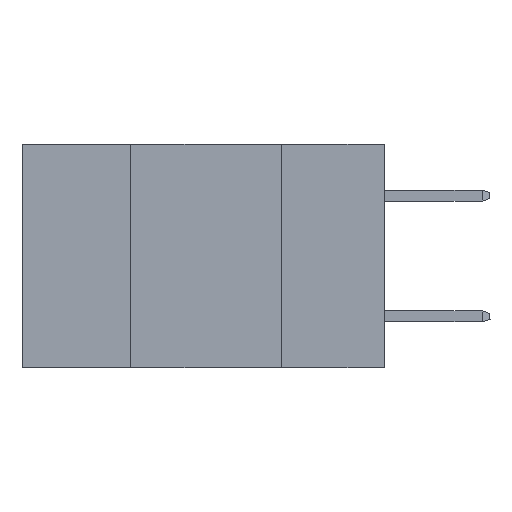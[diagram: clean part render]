
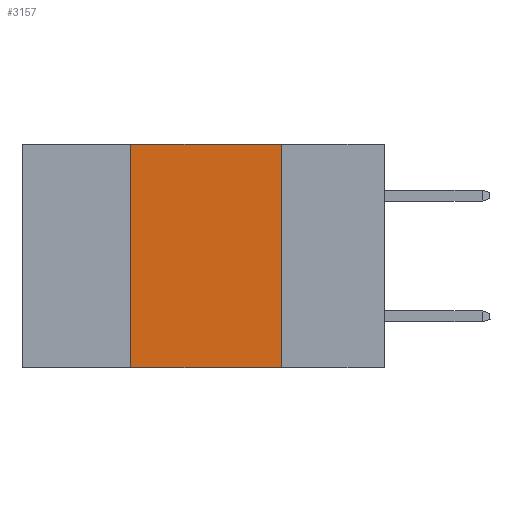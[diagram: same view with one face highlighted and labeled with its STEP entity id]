
A CAD part, left-side view. The second image highlights one B-rep face of the part: STEP entity #3157.
In plain terms, the highlighted planar face has unit normal (-1, 0, 0).
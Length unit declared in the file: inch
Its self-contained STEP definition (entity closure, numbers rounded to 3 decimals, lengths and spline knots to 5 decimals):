
#183 = CARTESIAN_POINT ( 'NONE',  ( 0., 0.42, 0. ) ) ;
#2216 = AXIS2_PLACEMENT_3D ( 'NONE', #23974, #23867, #23811 ) ;
#2990 = LINE ( 'NONE', #12541, #17729 ) ;
#3157 = ADVANCED_FACE ( 'NONE', ( #9960 ), #23886, .F. ) ;
#3906 = DIRECTION ( 'NONE',  ( 0., -1., 0. ) ) ;
#4594 = VERTEX_POINT ( 'NONE', #183 ) ;
#6420 = EDGE_LOOP ( 'NONE', ( #9777, #22170, #13093, #11470 ) ) ;
#8603 = CARTESIAN_POINT ( 'NONE',  ( 0., 0.42, -0.37 ) ) ;
#8774 = CARTESIAN_POINT ( 'NONE',  ( 0., 0.17, -0.37 ) ) ;
#9431 = CARTESIAN_POINT ( 'NONE',  ( 0., 0.42, -0.37 ) ) ;
#9777 = ORIENTED_EDGE ( 'NONE', *, *, #15619, .F. ) ;
#9898 = VECTOR ( 'NONE', #18606, 39.37008 ) ;
#9960 = FACE_OUTER_BOUND ( 'NONE', #6420, .T. ) ;
#10518 = EDGE_CURVE ( 'NONE', #12971, #4594, #18497, .T. ) ;
#11470 = ORIENTED_EDGE ( 'NONE', *, *, #19007, .T. ) ;
#12541 = CARTESIAN_POINT ( 'NONE',  ( 0., 0.6, -0.37 ) ) ;
#12971 = VERTEX_POINT ( 'NONE', #9431 ) ;
#13093 = ORIENTED_EDGE ( 'NONE', *, *, #10518, .F. ) ;
#14024 = VECTOR ( 'NONE', #20042, 39.37008 ) ;
#14466 = DIRECTION ( 'NONE',  ( 0., -1., 0. ) ) ;
#14797 = VERTEX_POINT ( 'NONE', #8774 ) ;
#15003 = LINE ( 'NONE', #24221, #9898 ) ;
#15619 = EDGE_CURVE ( 'NONE', #21280, #14797, #15003, .T. ) ;
#17705 = CARTESIAN_POINT ( 'NONE',  ( 0., 0.17, 0. ) ) ;
#17729 = VECTOR ( 'NONE', #14466, 39.37008 ) ;
#18497 = LINE ( 'NONE', #8603, #14024 ) ;
#18606 = DIRECTION ( 'NONE',  ( 0., 0., -1. ) ) ;
#19007 = EDGE_CURVE ( 'NONE', #12971, #14797, #2990, .T. ) ;
#20042 = DIRECTION ( 'NONE',  ( 0., 0., 1. ) ) ;
#20247 = LINE ( 'NONE', #23050, #24662 ) ;
#21280 = VERTEX_POINT ( 'NONE', #17705 ) ;
#21848 = EDGE_CURVE ( 'NONE', #4594, #21280, #20247, .T. ) ;
#22170 = ORIENTED_EDGE ( 'NONE', *, *, #21848, .F. ) ;
#23050 = CARTESIAN_POINT ( 'NONE',  ( 0., 0.6, 0. ) ) ;
#23811 = DIRECTION ( 'NONE',  ( 0., 0., -1. ) ) ;
#23867 = DIRECTION ( 'NONE',  ( 1., 0., 0. ) ) ;
#23886 = PLANE ( 'NONE',  #2216 ) ;
#23974 = CARTESIAN_POINT ( 'NONE',  ( 0., 0.6, 0. ) ) ;
#24221 = CARTESIAN_POINT ( 'NONE',  ( 0., 0.17, -0.37 ) ) ;
#24662 = VECTOR ( 'NONE', #3906, 39.37008 ) ;
